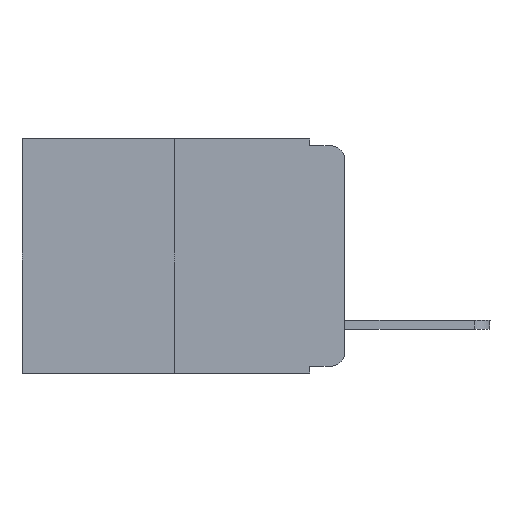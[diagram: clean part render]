
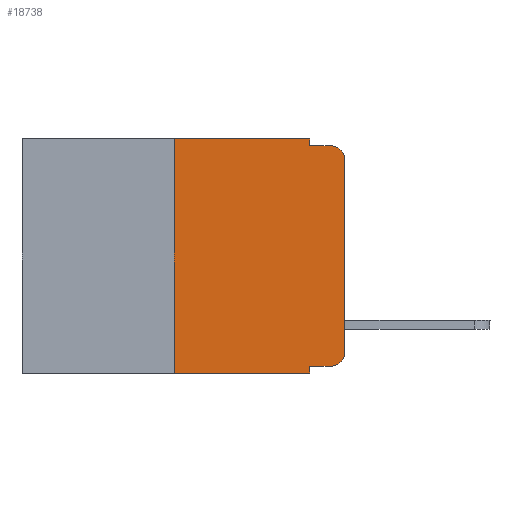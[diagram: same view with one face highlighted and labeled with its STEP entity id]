
A CAD part, left-side view. The second image highlights one B-rep face of the part: STEP entity #18738.
In plain terms, the highlighted planar face has unit normal (-1, 0, 0).
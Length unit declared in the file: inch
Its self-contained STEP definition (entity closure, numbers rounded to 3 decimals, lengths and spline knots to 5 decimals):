
#744 = CARTESIAN_POINT ( 'NONE',  ( 0., 0.473, 0. ) ) ;
#1089 = CARTESIAN_POINT ( 'NONE',  ( 0., 0.051, -0.343 ) ) ;
#1243 = DIRECTION ( 'NONE',  ( -1., 0., 0. ) ) ;
#1836 = EDGE_CURVE ( 'NONE', #3751, #14520, #23277, .T. ) ;
#2247 = VERTEX_POINT ( 'NONE', #18535 ) ;
#2725 = CIRCLE ( 'NONE', #7101, 0.02 ) ;
#2941 = LINE ( 'NONE', #12656, #8357 ) ;
#2955 = DIRECTION ( 'NONE',  ( 0., -1., 0. ) ) ;
#3061 = EDGE_CURVE ( 'NONE', #15883, #2247, #23270, .T. ) ;
#3090 = CARTESIAN_POINT ( 'NONE',  ( 0., 0.25, -0.343 ) ) ;
#3516 = VECTOR ( 'NONE', #11890, 39.37008 ) ;
#3751 = VERTEX_POINT ( 'NONE', #11667 ) ;
#4063 = CARTESIAN_POINT ( 'NONE',  ( 0., 0.473, -0.343 ) ) ;
#4365 = VECTOR ( 'NONE', #19275, 39.37008 ) ;
#4558 = CARTESIAN_POINT ( 'NONE',  ( 0., 0.051, 0. ) ) ;
#4638 = VECTOR ( 'NONE', #9242, 39.37008 ) ;
#5130 = VERTEX_POINT ( 'NONE', #3090 ) ;
#5719 = ORIENTED_EDGE ( 'NONE', *, *, #11238, .F. ) ;
#5841 = ORIENTED_EDGE ( 'NONE', *, *, #17972, .T. ) ;
#5938 = LINE ( 'NONE', #4063, #4365 ) ;
#5985 = CARTESIAN_POINT ( 'NONE',  ( 0., 0.02, -0.03 ) ) ;
#6018 = ORIENTED_EDGE ( 'NONE', *, *, #17786, .F. ) ;
#6157 = CARTESIAN_POINT ( 'NONE',  ( 0., 0., 0. ) ) ;
#6223 = PLANE ( 'NONE',  #22104 ) ;
#6421 = CARTESIAN_POINT ( 'NONE',  ( 0., 0.25, 0. ) ) ;
#6998 = LINE ( 'NONE', #10989, #4638 ) ;
#7101 = AXIS2_PLACEMENT_3D ( 'NONE', #5985, #21075, #17440 ) ;
#7968 = VERTEX_POINT ( 'NONE', #21447 ) ;
#8100 = LINE ( 'NONE', #12333, #10994 ) ;
#8221 = DIRECTION ( 'NONE',  ( 0., 0., 1. ) ) ;
#8357 = VECTOR ( 'NONE', #10417, 39.37008 ) ;
#8433 = LINE ( 'NONE', #4558, #11690 ) ;
#9081 = CARTESIAN_POINT ( 'NONE',  ( 0., 0.02, -0.313 ) ) ;
#9242 = DIRECTION ( 'NONE',  ( 0., -1., 0. ) ) ;
#9344 = CARTESIAN_POINT ( 'NONE',  ( 0., 0.02, -0.333 ) ) ;
#10094 = FACE_OUTER_BOUND ( 'NONE', #22826, .T. ) ;
#10417 = DIRECTION ( 'NONE',  ( 0., -1., 0. ) ) ;
#10524 = VERTEX_POINT ( 'NONE', #9344 ) ;
#10729 = ORIENTED_EDGE ( 'NONE', *, *, #3061, .F. ) ;
#10989 = CARTESIAN_POINT ( 'NONE',  ( 0., 0.051, -0.01 ) ) ;
#10994 = VECTOR ( 'NONE', #8221, 39.37008 ) ;
#11077 = DIRECTION ( 'NONE',  ( 0., 0., -1. ) ) ;
#11089 = ORIENTED_EDGE ( 'NONE', *, *, #21358, .T. ) ;
#11152 = EDGE_CURVE ( 'NONE', #5130, #20585, #5938, .T. ) ;
#11238 = EDGE_CURVE ( 'NONE', #20882, #15883, #2941, .T. ) ;
#11667 = CARTESIAN_POINT ( 'NONE',  ( 0., 0., -0.313 ) ) ;
#11690 = VECTOR ( 'NONE', #12177, 39.37008 ) ;
#11710 = ORIENTED_EDGE ( 'NONE', *, *, #1836, .T. ) ;
#11890 = DIRECTION ( 'NONE',  ( 0., 0., 1. ) ) ;
#12006 = CARTESIAN_POINT ( 'NONE',  ( 0., 0.051, 0. ) ) ;
#12177 = DIRECTION ( 'NONE',  ( 0., 0., -1. ) ) ;
#12333 = CARTESIAN_POINT ( 'NONE',  ( 0., 0.25, 0. ) ) ;
#12656 = CARTESIAN_POINT ( 'NONE',  ( 0., 0.473, 0. ) ) ;
#12694 = VECTOR ( 'NONE', #15865, 39.37008 ) ;
#13035 = CIRCLE ( 'NONE', #13776, 0.02 ) ;
#13776 = AXIS2_PLACEMENT_3D ( 'NONE', #9081, #1243, #11077 ) ;
#14520 = VERTEX_POINT ( 'NONE', #14552 ) ;
#14552 = CARTESIAN_POINT ( 'NONE',  ( 0., 0., -0.03 ) ) ;
#14706 = ORIENTED_EDGE ( 'NONE', *, *, #20937, .F. ) ;
#15070 = ORIENTED_EDGE ( 'NONE', *, *, #11152, .T. ) ;
#15504 = VERTEX_POINT ( 'NONE', #22750 ) ;
#15865 = DIRECTION ( 'NONE',  ( 0., 0., -1. ) ) ;
#15883 = VERTEX_POINT ( 'NONE', #20947 ) ;
#17440 = DIRECTION ( 'NONE',  ( 0., 0., -1. ) ) ;
#17686 = DIRECTION ( 'NONE',  ( 0., 0., -1. ) ) ;
#17771 = ORIENTED_EDGE ( 'NONE', *, *, #23204, .T. ) ;
#17786 = EDGE_CURVE ( 'NONE', #15504, #20585, #8433, .T. ) ;
#17972 = EDGE_CURVE ( 'NONE', #15504, #10524, #20024, .T. ) ;
#18485 = VECTOR ( 'NONE', #2955, 39.37008 ) ;
#18535 = CARTESIAN_POINT ( 'NONE',  ( 0., 0.051, -0.01 ) ) ;
#18738 = ADVANCED_FACE ( 'NONE', ( #10094 ), #6223, .F. ) ;
#19275 = DIRECTION ( 'NONE',  ( 0., -1., 0. ) ) ;
#19945 = EDGE_CURVE ( 'NONE', #5130, #20882, #8100, .T. ) ;
#20024 = LINE ( 'NONE', #22027, #18485 ) ;
#20585 = VERTEX_POINT ( 'NONE', #1089 ) ;
#20882 = VERTEX_POINT ( 'NONE', #6421 ) ;
#20937 = EDGE_CURVE ( 'NONE', #2247, #7968, #6998, .T. ) ;
#20947 = CARTESIAN_POINT ( 'NONE',  ( 0., 0.051, 0. ) ) ;
#21075 = DIRECTION ( 'NONE',  ( -1., 0., 0. ) ) ;
#21358 = EDGE_CURVE ( 'NONE', #10524, #3751, #13035, .T. ) ;
#21447 = CARTESIAN_POINT ( 'NONE',  ( 0., 0.02, -0.01 ) ) ;
#22027 = CARTESIAN_POINT ( 'NONE',  ( 0., 0.051, -0.333 ) ) ;
#22104 = AXIS2_PLACEMENT_3D ( 'NONE', #744, #23583, #17686 ) ;
#22750 = CARTESIAN_POINT ( 'NONE',  ( 0., 0.051, -0.333 ) ) ;
#22826 = EDGE_LOOP ( 'NONE', ( #11710, #17771, #14706, #10729, #5719, #24284, #15070, #6018, #5841, #11089 ) ) ;
#23204 = EDGE_CURVE ( 'NONE', #14520, #7968, #2725, .T. ) ;
#23270 = LINE ( 'NONE', #12006, #12694 ) ;
#23277 = LINE ( 'NONE', #6157, #3516 ) ;
#23583 = DIRECTION ( 'NONE',  ( 1., 0., 0. ) ) ;
#24284 = ORIENTED_EDGE ( 'NONE', *, *, #19945, .F. ) ;
